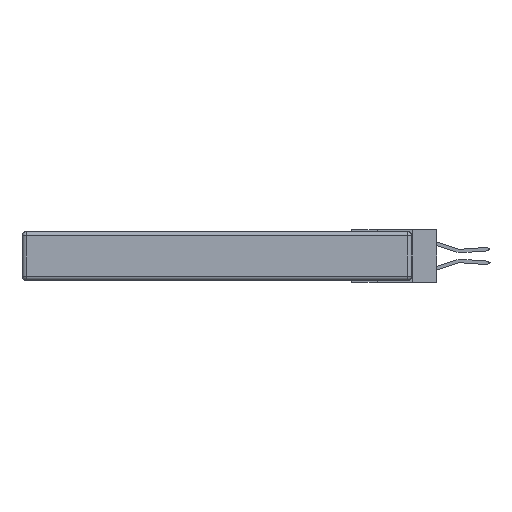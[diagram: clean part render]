
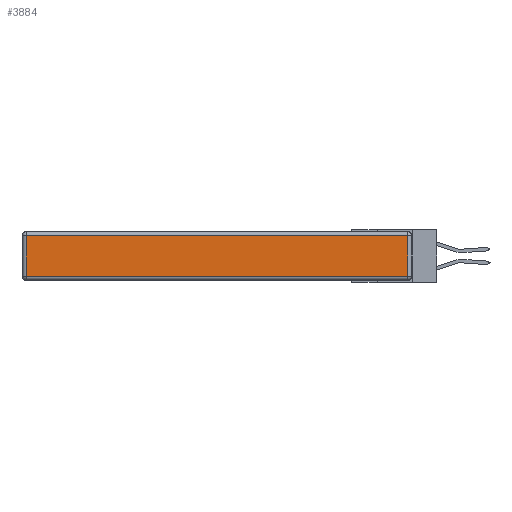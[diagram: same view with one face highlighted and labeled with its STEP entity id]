
A CAD part, left-side view. The second image highlights one B-rep face of the part: STEP entity #3884.
In plain terms, the highlighted planar face has unit normal (-1, 0, 0).
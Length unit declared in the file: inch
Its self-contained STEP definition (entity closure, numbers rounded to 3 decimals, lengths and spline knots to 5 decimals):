
#423 = LINE ( 'NONE', #22307, #17545 ) ;
#804 = VERTEX_POINT ( 'NONE', #25598 ) ;
#1246 = CARTESIAN_POINT ( 'NONE',  ( 0., 2.72, -0.343 ) ) ;
#1405 = LINE ( 'NONE', #1246, #11429 ) ;
#2727 = ORIENTED_EDGE ( 'NONE', *, *, #4950, .T. ) ;
#3304 = EDGE_CURVE ( 'NONE', #17698, #10907, #423, .T. ) ;
#3884 = ADVANCED_FACE ( 'NONE', ( #16636 ), #14648, .T. ) ;
#4014 = ORIENTED_EDGE ( 'NONE', *, *, #3304, .T. ) ;
#4410 = DIRECTION ( 'NONE',  ( 0., 1., 0. ) ) ;
#4632 = DIRECTION ( 'NONE',  ( 0., 0., 1. ) ) ;
#4714 = VECTOR ( 'NONE', #5983, 39.37008 ) ;
#4799 = DIRECTION ( 'NONE',  ( -1., 0., 0. ) ) ;
#4890 = CARTESIAN_POINT ( 'NONE',  ( 0., 0.03, -0.03 ) ) ;
#4950 = EDGE_CURVE ( 'NONE', #18333, #17698, #14100, .T. ) ;
#5983 = DIRECTION ( 'NONE',  ( 0., 0., 1. ) ) ;
#6736 = VECTOR ( 'NONE', #17279, 39.37008 ) ;
#10907 = VERTEX_POINT ( 'NONE', #23332 ) ;
#11429 = VECTOR ( 'NONE', #23346, 39.37008 ) ;
#12121 = CARTESIAN_POINT ( 'NONE',  ( 0., 0.03, -0.343 ) ) ;
#13317 = LINE ( 'NONE', #19035, #6736 ) ;
#13993 = EDGE_CURVE ( 'NONE', #10907, #804, #1405, .T. ) ;
#14100 = LINE ( 'NONE', #12121, #4714 ) ;
#14648 = PLANE ( 'NONE',  #21314 ) ;
#15156 = ORIENTED_EDGE ( 'NONE', *, *, #13993, .T. ) ;
#16636 = FACE_OUTER_BOUND ( 'NONE', #18255, .T. ) ;
#17279 = DIRECTION ( 'NONE',  ( 0., -1., 0. ) ) ;
#17545 = VECTOR ( 'NONE', #4410, 39.37008 ) ;
#17698 = VERTEX_POINT ( 'NONE', #4890 ) ;
#18255 = EDGE_LOOP ( 'NONE', ( #20762, #2727, #4014, #15156 ) ) ;
#18333 = VERTEX_POINT ( 'NONE', #24865 ) ;
#18826 = CARTESIAN_POINT ( 'NONE',  ( 0., 0., -0.343 ) ) ;
#19035 = CARTESIAN_POINT ( 'NONE',  ( 0., 0., -0.313 ) ) ;
#20762 = ORIENTED_EDGE ( 'NONE', *, *, #21942, .T. ) ;
#21314 = AXIS2_PLACEMENT_3D ( 'NONE', #18826, #4799, #4632 ) ;
#21942 = EDGE_CURVE ( 'NONE', #804, #18333, #13317, .T. ) ;
#22307 = CARTESIAN_POINT ( 'NONE',  ( 0., 2.75, -0.03 ) ) ;
#23332 = CARTESIAN_POINT ( 'NONE',  ( 0., 2.72, -0.03 ) ) ;
#23346 = DIRECTION ( 'NONE',  ( 0., 0., -1. ) ) ;
#24865 = CARTESIAN_POINT ( 'NONE',  ( 0., 0.03, -0.313 ) ) ;
#25598 = CARTESIAN_POINT ( 'NONE',  ( 0., 2.72, -0.313 ) ) ;
